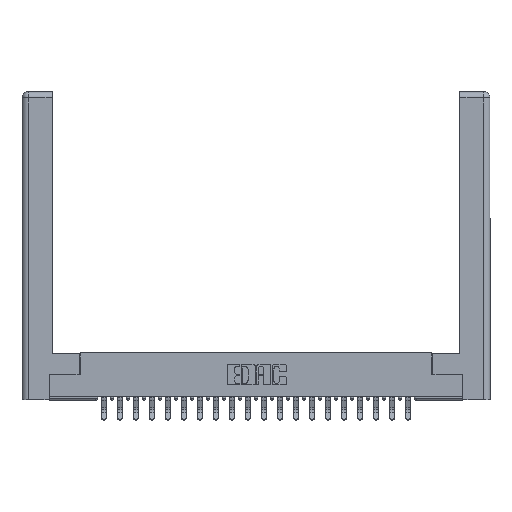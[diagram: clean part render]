
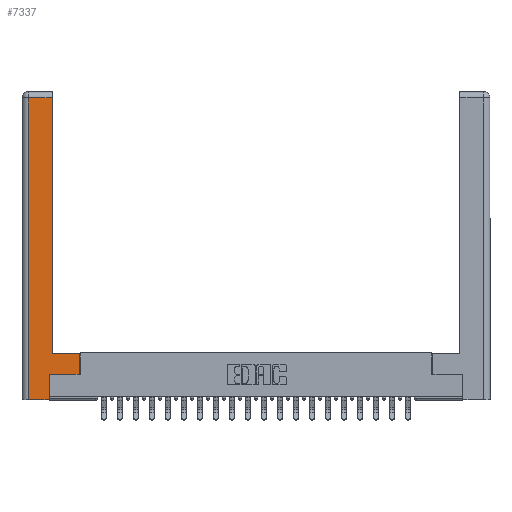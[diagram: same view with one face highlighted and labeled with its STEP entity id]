
A CAD part, top view. The second image highlights one B-rep face of the part: STEP entity #7337.
In plain terms, the highlighted planar face has unit normal (0, 0, 1).
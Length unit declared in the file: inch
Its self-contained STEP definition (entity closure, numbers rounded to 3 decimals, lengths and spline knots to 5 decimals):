
#268 = VERTEX_POINT ( 'NONE', #17336 ) ;
#318 = CARTESIAN_POINT ( 'NONE',  ( 0.565, 0.45, 0. ) ) ;
#370 = CARTESIAN_POINT ( 'NONE',  ( 0.0615, 0., 0. ) ) ;
#378 = CARTESIAN_POINT ( 'NONE',  ( 0.565, 0.245, 0. ) ) ;
#1394 = EDGE_CURVE ( 'NONE', #22766, #4773, #5338, .T. ) ;
#1457 = EDGE_CURVE ( 'NONE', #14777, #22766, #25713, .T. ) ;
#2479 = LINE ( 'NONE', #25595, #10725 ) ;
#2766 = CARTESIAN_POINT ( 'NONE',  ( 0.265, 0.245, 0. ) ) ;
#2779 = LINE ( 'NONE', #2766, #18879 ) ;
#2844 = LINE ( 'NONE', #18992, #21240 ) ;
#2863 = EDGE_CURVE ( 'NONE', #4773, #26552, #5287, .T. ) ;
#3552 = CARTESIAN_POINT ( 'NONE',  ( 0.565, 0.45, 0. ) ) ;
#4013 = DIRECTION ( 'NONE',  ( 1., 0., 0. ) ) ;
#4773 = VERTEX_POINT ( 'NONE', #13172 ) ;
#5287 = LINE ( 'NONE', #12640, #25344 ) ;
#5338 = LINE ( 'NONE', #25616, #16547 ) ;
#5382 = CARTESIAN_POINT ( 'NONE',  ( 0.565, 0.245, 0. ) ) ;
#5391 = EDGE_CURVE ( 'NONE', #18869, #268, #2844, .T. ) ;
#5413 = ORIENTED_EDGE ( 'NONE', *, *, #1394, .T. ) ;
#5530 = ORIENTED_EDGE ( 'NONE', *, *, #26152, .T. ) ;
#5950 = ORIENTED_EDGE ( 'NONE', *, *, #19916, .T. ) ;
#6107 = ORIENTED_EDGE ( 'NONE', *, *, #1457, .T. ) ;
#6711 = EDGE_CURVE ( 'NONE', #268, #24614, #2779, .T. ) ;
#6733 = LINE ( 'NONE', #378, #24456 ) ;
#7196 = ORIENTED_EDGE ( 'NONE', *, *, #5391, .T. ) ;
#7337 = ADVANCED_FACE ( 'NONE', ( #15665 ), #25768, .F. ) ;
#8019 = LINE ( 'NONE', #370, #20485 ) ;
#8101 = VERTEX_POINT ( 'NONE', #14313 ) ;
#8700 = DIRECTION ( 'NONE',  ( 0., 0., -1. ) ) ;
#8843 = DIRECTION ( 'NONE',  ( 1., 0., 0. ) ) ;
#10725 = VECTOR ( 'NONE', #17338, 39.37008 ) ;
#11054 = DIRECTION ( 'NONE',  ( 0., -1., 0. ) ) ;
#12541 = DIRECTION ( 'NONE',  ( 0., 1., 0. ) ) ;
#12640 = CARTESIAN_POINT ( 'NONE',  ( 0.295, 3., 0. ) ) ;
#13025 = DIRECTION ( 'NONE',  ( -1., 0., 0. ) ) ;
#13172 = CARTESIAN_POINT ( 'NONE',  ( 0.295, 0.45, 0. ) ) ;
#13357 = ORIENTED_EDGE ( 'NONE', *, *, #6711, .T. ) ;
#14313 = CARTESIAN_POINT ( 'NONE',  ( 0.0615, 2.94, 0. ) ) ;
#14777 = VERTEX_POINT ( 'NONE', #5382 ) ;
#14866 = DIRECTION ( 'NONE',  ( 0., 1., 0. ) ) ;
#15041 = ORIENTED_EDGE ( 'NONE', *, *, #17339, .T. ) ;
#15665 = FACE_OUTER_BOUND ( 'NONE', #22630, .T. ) ;
#15906 = ORIENTED_EDGE ( 'NONE', *, *, #2863, .T. ) ;
#16247 = CARTESIAN_POINT ( 'NONE',  ( 0.0615, 0., 0. ) ) ;
#16547 = VECTOR ( 'NONE', #13025, 39.37008 ) ;
#16970 = DIRECTION ( 'NONE',  ( -1., 0., 0. ) ) ;
#17336 = CARTESIAN_POINT ( 'NONE',  ( 0.265, 0., 0. ) ) ;
#17338 = DIRECTION ( 'NONE',  ( -1., 0., 0. ) ) ;
#17339 = EDGE_CURVE ( 'NONE', #26552, #8101, #2479, .T. ) ;
#18869 = VERTEX_POINT ( 'NONE', #16247 ) ;
#18879 = VECTOR ( 'NONE', #19377, 39.37008 ) ;
#18992 = CARTESIAN_POINT ( 'NONE',  ( 0.265, 0., 0. ) ) ;
#19377 = DIRECTION ( 'NONE',  ( 0., 1., 0. ) ) ;
#19916 = EDGE_CURVE ( 'NONE', #8101, #18869, #8019, .T. ) ;
#20485 = VECTOR ( 'NONE', #11054, 39.37008 ) ;
#21240 = VECTOR ( 'NONE', #4013, 39.37008 ) ;
#21437 = VECTOR ( 'NONE', #14866, 39.37008 ) ;
#22373 = CARTESIAN_POINT ( 'NONE',  ( 0.295, 2.94, 0. ) ) ;
#22630 = EDGE_LOOP ( 'NONE', ( #15906, #15041, #5950, #7196, #13357, #5530, #6107, #5413 ) ) ;
#22766 = VERTEX_POINT ( 'NONE', #3552 ) ;
#23544 = CARTESIAN_POINT ( 'NONE',  ( 0., 0., 0. ) ) ;
#24322 = CARTESIAN_POINT ( 'NONE',  ( 0.265, 0.245, 0. ) ) ;
#24456 = VECTOR ( 'NONE', #8843, 39.37008 ) ;
#24564 = AXIS2_PLACEMENT_3D ( 'NONE', #23544, #8700, #16970 ) ;
#24614 = VERTEX_POINT ( 'NONE', #24322 ) ;
#25344 = VECTOR ( 'NONE', #12541, 39.37008 ) ;
#25595 = CARTESIAN_POINT ( 'NONE',  ( 0.0615, 2.94, 0. ) ) ;
#25616 = CARTESIAN_POINT ( 'NONE',  ( 0.295, 0.45, 0. ) ) ;
#25713 = LINE ( 'NONE', #318, #21437 ) ;
#25768 = PLANE ( 'NONE',  #24564 ) ;
#26152 = EDGE_CURVE ( 'NONE', #24614, #14777, #6733, .T. ) ;
#26552 = VERTEX_POINT ( 'NONE', #22373 ) ;
